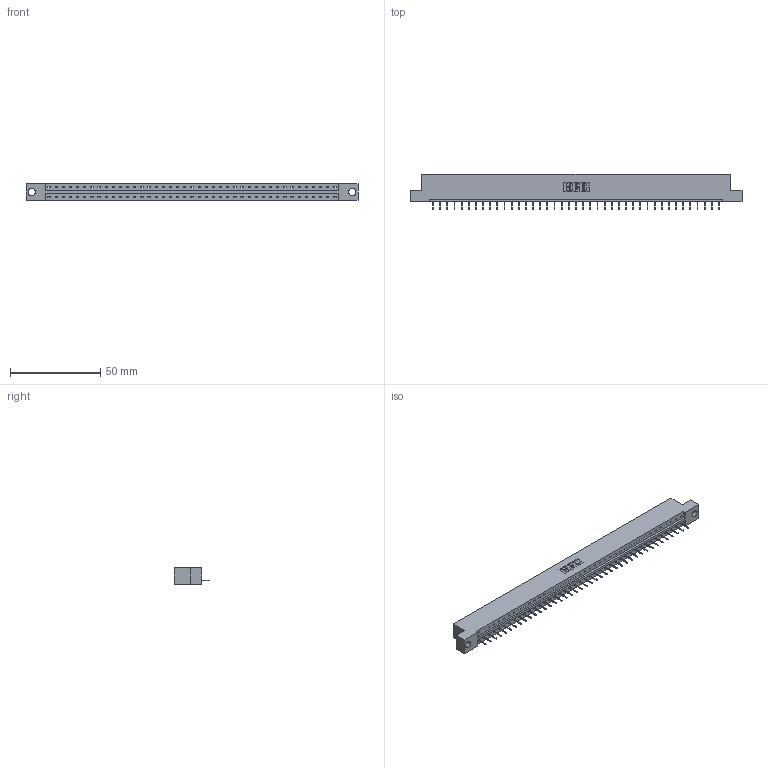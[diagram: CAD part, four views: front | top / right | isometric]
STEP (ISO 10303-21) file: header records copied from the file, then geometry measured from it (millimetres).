
FILE_DESCRIPTION (( 'STEP AP203' ), '1' );
FILE_NAME ('833-041-524-104.STEP', '2020-06-03T19:00:07', ( '' ), ( '' ), 'SwSTEP 2.0', 'SolidWorks 2020', '' );
FILE_SCHEMA (( 'CONFIG_CONTROL_DESIGN' ));
Length unit declared in the file: inch
Products named in the file (3): 345-292-001_345-293-124; 833 Part_Flush - .156 Dia - TH; 833-041-524-104
Assembly tree (42 placements, depth 2):
  833-041-524-104
    833 Part_Flush - .156 Dia - TH
    345-292-001_345-293-124  x41
Bounding box: 184 x 19.69 x 9.4 mm (x, y, z)
Volume: 18256.9 mm3; surface area: 18985.9 mm2
Topology: 42 solids, 42 shells, 2656 faces, 7691 edges, 4962 vertices
Faces by surface type: plane 2038, cylinder 618
Entity records: 25271 total; most frequent: CARTESIAN_POINT 4365, ORIENTED_EDGE 4342, DIRECTION 3685, EDGE_CURVE 2171, LINE 2047, VECTOR 2047, VERTEX_POINT 1442, AXIS2_PLACEMENT_3D 819
